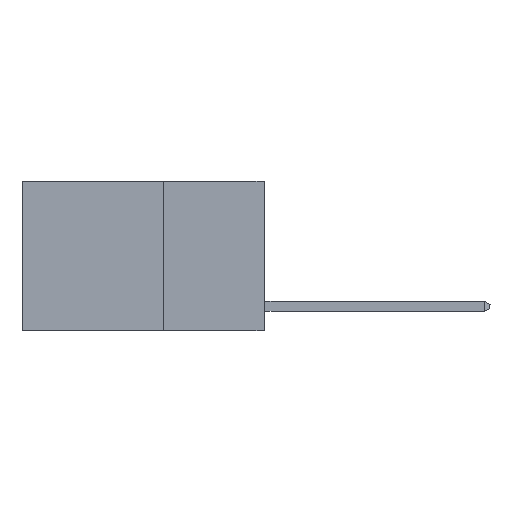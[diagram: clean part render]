
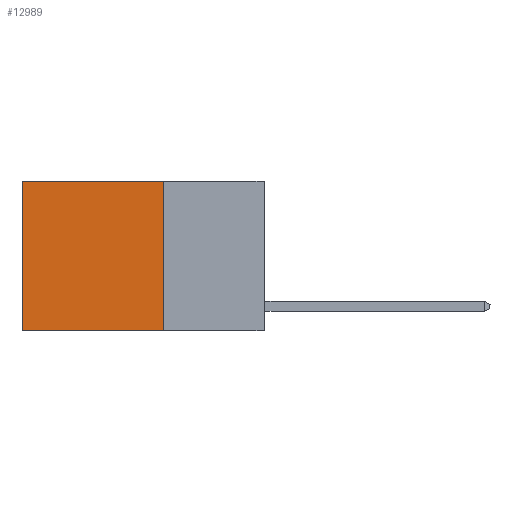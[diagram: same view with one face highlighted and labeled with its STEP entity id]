
A CAD part, left-side view. The second image highlights one B-rep face of the part: STEP entity #12989.
In plain terms, the highlighted planar face has unit normal (-1, 0, 0).
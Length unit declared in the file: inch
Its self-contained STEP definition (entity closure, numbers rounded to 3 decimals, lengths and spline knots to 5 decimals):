
#480 = DIRECTION ( 'NONE',  ( 1., 0., 0. ) ) ;
#1083 = VERTEX_POINT ( 'NONE', #14637 ) ;
#1119 = CARTESIAN_POINT ( 'NONE',  ( 0.2625, 0.25, -0.37 ) ) ;
#2982 = VECTOR ( 'NONE', #3600, 39.37008 ) ;
#3600 = DIRECTION ( 'NONE',  ( 0., 1., 0. ) ) ;
#3796 = DIRECTION ( 'NONE',  ( 0., 0., -1. ) ) ;
#3820 = VERTEX_POINT ( 'NONE', #1119 ) ;
#3859 = VERTEX_POINT ( 'NONE', #4985 ) ;
#4333 = EDGE_CURVE ( 'NONE', #1083, #12676, #7475, .T. ) ;
#4985 = CARTESIAN_POINT ( 'NONE',  ( 0.2625, 0.6, -0.37 ) ) ;
#5189 = LINE ( 'NONE', #11149, #2982 ) ;
#5505 = PLANE ( 'NONE',  #9720 ) ;
#5560 = CARTESIAN_POINT ( 'NONE',  ( 0.2625, 0.25, 0. ) ) ;
#7103 = CARTESIAN_POINT ( 'NONE',  ( 0.2625, 0.6, 0. ) ) ;
#7290 = LINE ( 'NONE', #10587, #13915 ) ;
#7475 = LINE ( 'NONE', #9354, #9495 ) ;
#7496 = CARTESIAN_POINT ( 'NONE',  ( 0.2625, 0.25, 0. ) ) ;
#8028 = ORIENTED_EDGE ( 'NONE', *, *, #11691, .F. ) ;
#8674 = EDGE_CURVE ( 'NONE', #3820, #3859, #5189, .T. ) ;
#9306 = DIRECTION ( 'NONE',  ( 0., 0., -1. ) ) ;
#9354 = CARTESIAN_POINT ( 'NONE',  ( 0.2625, 0.25, 0. ) ) ;
#9495 = VECTOR ( 'NONE', #10575, 39.37008 ) ;
#9715 = EDGE_LOOP ( 'NONE', ( #13959, #9759, #8028, #13518 ) ) ;
#9720 = AXIS2_PLACEMENT_3D ( 'NONE', #5560, #480, #9306 ) ;
#9759 = ORIENTED_EDGE ( 'NONE', *, *, #8674, .F. ) ;
#10157 = LINE ( 'NONE', #7496, #15960 ) ;
#10575 = DIRECTION ( 'NONE',  ( 0., 1., 0. ) ) ;
#10587 = CARTESIAN_POINT ( 'NONE',  ( 0.2625, 0.6, 0. ) ) ;
#11149 = CARTESIAN_POINT ( 'NONE',  ( 0.2625, 0.25, -0.37 ) ) ;
#11691 = EDGE_CURVE ( 'NONE', #1083, #3820, #10157, .T. ) ;
#11861 = DIRECTION ( 'NONE',  ( 0., 0., -1. ) ) ;
#12676 = VERTEX_POINT ( 'NONE', #7103 ) ;
#12989 = ADVANCED_FACE ( 'NONE', ( #13320 ), #5505, .F. ) ;
#13067 = EDGE_CURVE ( 'NONE', #12676, #3859, #7290, .T. ) ;
#13320 = FACE_OUTER_BOUND ( 'NONE', #9715, .T. ) ;
#13518 = ORIENTED_EDGE ( 'NONE', *, *, #4333, .T. ) ;
#13915 = VECTOR ( 'NONE', #11861, 39.37008 ) ;
#13959 = ORIENTED_EDGE ( 'NONE', *, *, #13067, .T. ) ;
#14637 = CARTESIAN_POINT ( 'NONE',  ( 0.2625, 0.25, 0. ) ) ;
#15960 = VECTOR ( 'NONE', #3796, 39.37008 ) ;
